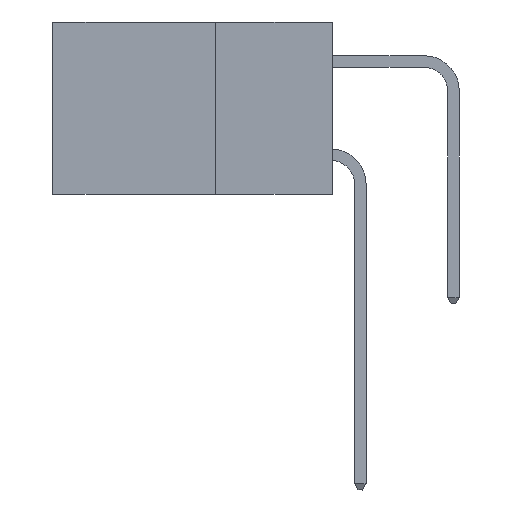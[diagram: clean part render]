
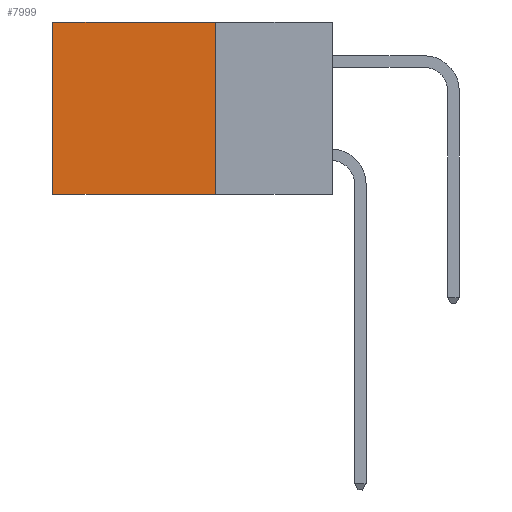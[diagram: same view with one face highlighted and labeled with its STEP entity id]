
A CAD part, left-side view. The second image highlights one B-rep face of the part: STEP entity #7999.
In plain terms, the highlighted planar face has unit normal (-1, 0, 0).
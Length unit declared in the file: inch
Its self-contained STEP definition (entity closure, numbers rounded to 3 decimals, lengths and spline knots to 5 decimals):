
#29 = VECTOR ( 'NONE', #7881, 39.37008 ) ;
#764 = VERTEX_POINT ( 'NONE', #1041 ) ;
#1041 = CARTESIAN_POINT ( 'NONE',  ( 0.2615, 0.6, 0. ) ) ;
#1572 = CARTESIAN_POINT ( 'NONE',  ( 0.2615, 0.25, 0. ) ) ;
#2198 = LINE ( 'NONE', #4340, #10960 ) ;
#2540 = LINE ( 'NONE', #8956, #29 ) ;
#2720 = ORIENTED_EDGE ( 'NONE', *, *, #6734, .F. ) ;
#3190 = VERTEX_POINT ( 'NONE', #7752 ) ;
#3631 = CARTESIAN_POINT ( 'NONE',  ( 0.2615, 0.25, -0.37 ) ) ;
#3642 = DIRECTION ( 'NONE',  ( 0., 0., -1. ) ) ;
#4340 = CARTESIAN_POINT ( 'NONE',  ( 0.2615, 0.25, -0.37 ) ) ;
#4781 = PLANE ( 'NONE',  #6421 ) ;
#5151 = ORIENTED_EDGE ( 'NONE', *, *, #8653, .T. ) ;
#5187 = LINE ( 'NONE', #5256, #12333 ) ;
#5256 = CARTESIAN_POINT ( 'NONE',  ( 0.2615, 0.25, 0. ) ) ;
#5358 = ORIENTED_EDGE ( 'NONE', *, *, #8217, .F. ) ;
#5619 = ORIENTED_EDGE ( 'NONE', *, *, #5912, .T. ) ;
#5775 = FACE_OUTER_BOUND ( 'NONE', #8707, .T. ) ;
#5912 = EDGE_CURVE ( 'NONE', #764, #9867, #10465, .T. ) ;
#6421 = AXIS2_PLACEMENT_3D ( 'NONE', #3631, #8048, #12387 ) ;
#6734 = EDGE_CURVE ( 'NONE', #3190, #9867, #2540, .T. ) ;
#7752 = CARTESIAN_POINT ( 'NONE',  ( 0.2615, 0.25, -0.37 ) ) ;
#7881 = DIRECTION ( 'NONE',  ( 0., 1., 0. ) ) ;
#7999 = ADVANCED_FACE ( 'NONE', ( #5775 ), #4781, .F. ) ;
#8048 = DIRECTION ( 'NONE',  ( 1., 0., 0. ) ) ;
#8217 = EDGE_CURVE ( 'NONE', #12148, #3190, #2198, .T. ) ;
#8653 = EDGE_CURVE ( 'NONE', #12148, #764, #5187, .T. ) ;
#8707 = EDGE_LOOP ( 'NONE', ( #5619, #2720, #5358, #5151 ) ) ;
#8956 = CARTESIAN_POINT ( 'NONE',  ( 0.2615, 0.25, -0.37 ) ) ;
#9867 = VERTEX_POINT ( 'NONE', #10371 ) ;
#10371 = CARTESIAN_POINT ( 'NONE',  ( 0.2615, 0.6, -0.37 ) ) ;
#10465 = LINE ( 'NONE', #13394, #10480 ) ;
#10480 = VECTOR ( 'NONE', #3642, 39.37008 ) ;
#10934 = DIRECTION ( 'NONE',  ( 0., 1., 0. ) ) ;
#10960 = VECTOR ( 'NONE', #12011, 39.37008 ) ;
#12011 = DIRECTION ( 'NONE',  ( 0., 0., -1. ) ) ;
#12148 = VERTEX_POINT ( 'NONE', #1572 ) ;
#12333 = VECTOR ( 'NONE', #10934, 39.37008 ) ;
#12387 = DIRECTION ( 'NONE',  ( 0., 0., -1. ) ) ;
#13394 = CARTESIAN_POINT ( 'NONE',  ( 0.2615, 0.6, -0.37 ) ) ;
